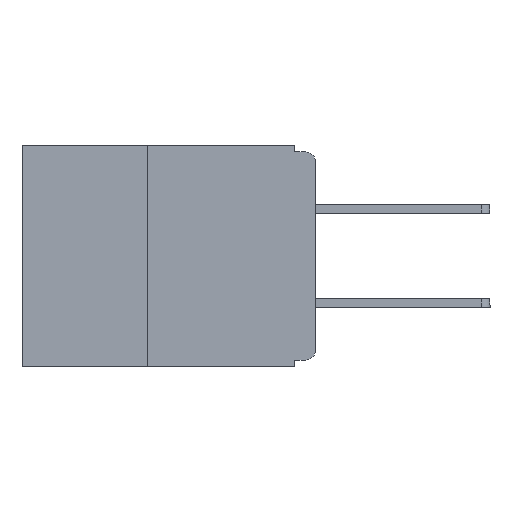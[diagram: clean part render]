
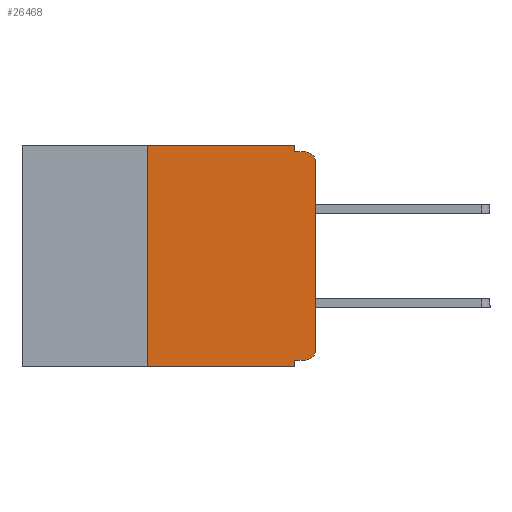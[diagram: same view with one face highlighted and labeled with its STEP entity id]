
A CAD part, left-side view. The second image highlights one B-rep face of the part: STEP entity #26468.
In plain terms, the highlighted planar face has unit normal (-1, 0, 0).
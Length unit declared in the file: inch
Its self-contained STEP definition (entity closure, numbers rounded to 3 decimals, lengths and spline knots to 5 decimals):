
#85 = ORIENTED_EDGE ( 'NONE', *, *, #14506, .T. ) ;
#166 = VERTEX_POINT ( 'NONE', #28376 ) ;
#224 = CARTESIAN_POINT ( 'NONE',  ( 0., 0., -0.305 ) ) ;
#712 = DIRECTION ( 'NONE',  ( 0., 1., 0. ) ) ;
#747 = CARTESIAN_POINT ( 'NONE',  ( 0., 0.031, -0.01 ) ) ;
#1453 = ORIENTED_EDGE ( 'NONE', *, *, #11683, .F. ) ;
#1948 = PLANE ( 'NONE',  #21761 ) ;
#2184 = VECTOR ( 'NONE', #2680, 39.37008 ) ;
#2245 = DIRECTION ( 'NONE',  ( 0., 0., -1. ) ) ;
#2580 = EDGE_CURVE ( 'NONE', #22790, #3437, #18989, .T. ) ;
#2680 = DIRECTION ( 'NONE',  ( 0., -1., 0. ) ) ;
#3003 = CARTESIAN_POINT ( 'NONE',  ( 0., 0., -0.01 ) ) ;
#3088 = CARTESIAN_POINT ( 'NONE',  ( 0., 0.015, -0.025 ) ) ;
#3130 = AXIS2_PLACEMENT_3D ( 'NONE', #3088, #20841, #5695 ) ;
#3437 = VERTEX_POINT ( 'NONE', #28913 ) ;
#4421 = DIRECTION ( 'NONE',  ( 0., -1., 0. ) ) ;
#5052 = EDGE_CURVE ( 'NONE', #12701, #13752, #29052, .T. ) ;
#5695 = DIRECTION ( 'NONE',  ( 0., 0., -1. ) ) ;
#6307 = LINE ( 'NONE', #10856, #25606 ) ;
#6633 = CARTESIAN_POINT ( 'NONE',  ( 0., 0., 0. ) ) ;
#7057 = CARTESIAN_POINT ( 'NONE',  ( 0., 0.437, 0. ) ) ;
#7106 = EDGE_CURVE ( 'NONE', #21183, #12701, #30797, .T. ) ;
#7148 = DIRECTION ( 'NONE',  ( 0., 0., -1. ) ) ;
#7344 = EDGE_CURVE ( 'NONE', #7995, #19113, #16431, .T. ) ;
#7995 = VERTEX_POINT ( 'NONE', #28814 ) ;
#9677 = CARTESIAN_POINT ( 'NONE',  ( 0., 0.031, -0.33 ) ) ;
#10053 = CARTESIAN_POINT ( 'NONE',  ( 0., 0., -0.025 ) ) ;
#10112 = CARTESIAN_POINT ( 'NONE',  ( 0., 0.031, 0. ) ) ;
#10478 = VERTEX_POINT ( 'NONE', #9677 ) ;
#10856 = CARTESIAN_POINT ( 'NONE',  ( 0., 0.031, -0.33 ) ) ;
#11139 = FACE_OUTER_BOUND ( 'NONE', #27347, .T. ) ;
#11315 = DIRECTION ( 'NONE',  ( -1., 0., 0. ) ) ;
#11510 = VECTOR ( 'NONE', #24477, 39.37008 ) ;
#11683 = EDGE_CURVE ( 'NONE', #3437, #21183, #17261, .T. ) ;
#12317 = CIRCLE ( 'NONE', #3130, 0.015 ) ;
#12701 = VERTEX_POINT ( 'NONE', #747 ) ;
#12939 = ORIENTED_EDGE ( 'NONE', *, *, #2580, .F. ) ;
#13605 = VERTEX_POINT ( 'NONE', #10053 ) ;
#13752 = VERTEX_POINT ( 'NONE', #20709 ) ;
#14092 = EDGE_CURVE ( 'NONE', #19113, #13605, #32208, .T. ) ;
#14506 = EDGE_CURVE ( 'NONE', #13605, #13752, #12317, .T. ) ;
#16039 = VECTOR ( 'NONE', #2245, 39.37008 ) ;
#16116 = ORIENTED_EDGE ( 'NONE', *, *, #5052, .F. ) ;
#16431 = CIRCLE ( 'NONE', #29182, 0.015 ) ;
#16510 = ORIENTED_EDGE ( 'NONE', *, *, #27618, .T. ) ;
#16770 = ORIENTED_EDGE ( 'NONE', *, *, #21967, .F. ) ;
#17261 = LINE ( 'NONE', #7057, #29695 ) ;
#17547 = CARTESIAN_POINT ( 'NONE',  ( 0., 0.25, -0.33 ) ) ;
#18254 = VECTOR ( 'NONE', #31711, 39.37008 ) ;
#18989 = LINE ( 'NONE', #24523, #11510 ) ;
#19113 = VERTEX_POINT ( 'NONE', #224 ) ;
#19587 = ORIENTED_EDGE ( 'NONE', *, *, #7344, .T. ) ;
#19725 = CARTESIAN_POINT ( 'NONE',  ( 0., 0.437, 0. ) ) ;
#20709 = CARTESIAN_POINT ( 'NONE',  ( 0., 0.015, -0.01 ) ) ;
#20717 = ORIENTED_EDGE ( 'NONE', *, *, #21379, .F. ) ;
#20841 = DIRECTION ( 'NONE',  ( -1., 0., 0. ) ) ;
#20949 = ORIENTED_EDGE ( 'NONE', *, *, #7106, .F. ) ;
#21183 = VERTEX_POINT ( 'NONE', #10112 ) ;
#21379 = EDGE_CURVE ( 'NONE', #166, #10478, #6307, .T. ) ;
#21733 = CARTESIAN_POINT ( 'NONE',  ( 0., 0.437, -0.33 ) ) ;
#21761 = AXIS2_PLACEMENT_3D ( 'NONE', #19725, #22236, #7148 ) ;
#21967 = EDGE_CURVE ( 'NONE', #7995, #166, #30240, .T. ) ;
#22111 = ORIENTED_EDGE ( 'NONE', *, *, #14092, .T. ) ;
#22236 = DIRECTION ( 'NONE',  ( 1., 0., 0. ) ) ;
#22790 = VERTEX_POINT ( 'NONE', #17547 ) ;
#23648 = VECTOR ( 'NONE', #712, 39.37008 ) ;
#24477 = DIRECTION ( 'NONE',  ( 0., 0., 1. ) ) ;
#24523 = CARTESIAN_POINT ( 'NONE',  ( 0., 0.25, -0.33 ) ) ;
#25271 = LINE ( 'NONE', #21733, #31041 ) ;
#25606 = VECTOR ( 'NONE', #28297, 39.37008 ) ;
#25996 = CARTESIAN_POINT ( 'NONE',  ( 0., 0., -0.32 ) ) ;
#26358 = CARTESIAN_POINT ( 'NONE',  ( 0., 0.015, -0.305 ) ) ;
#26468 = ADVANCED_FACE ( 'NONE', ( #11139 ), #1948, .F. ) ;
#27347 = EDGE_LOOP ( 'NONE', ( #22111, #85, #16116, #20949, #1453, #12939, #16510, #20717, #16770, #19587 ) ) ;
#27618 = EDGE_CURVE ( 'NONE', #22790, #10478, #25271, .T. ) ;
#28297 = DIRECTION ( 'NONE',  ( 0., 0., -1. ) ) ;
#28376 = CARTESIAN_POINT ( 'NONE',  ( 0., 0.031, -0.32 ) ) ;
#28814 = CARTESIAN_POINT ( 'NONE',  ( 0., 0.015, -0.32 ) ) ;
#28853 = DIRECTION ( 'NONE',  ( 0., 0., -1. ) ) ;
#28913 = CARTESIAN_POINT ( 'NONE',  ( 0., 0.25, 0. ) ) ;
#29052 = LINE ( 'NONE', #3003, #2184 ) ;
#29182 = AXIS2_PLACEMENT_3D ( 'NONE', #26358, #11315, #28853 ) ;
#29695 = VECTOR ( 'NONE', #4421, 39.37008 ) ;
#30240 = LINE ( 'NONE', #25996, #23648 ) ;
#30797 = LINE ( 'NONE', #32362, #16039 ) ;
#31041 = VECTOR ( 'NONE', #31701, 39.37008 ) ;
#31701 = DIRECTION ( 'NONE',  ( 0., -1., 0. ) ) ;
#31711 = DIRECTION ( 'NONE',  ( 0., 0., 1. ) ) ;
#32208 = LINE ( 'NONE', #6633, #18254 ) ;
#32362 = CARTESIAN_POINT ( 'NONE',  ( 0., 0.031, 0. ) ) ;
